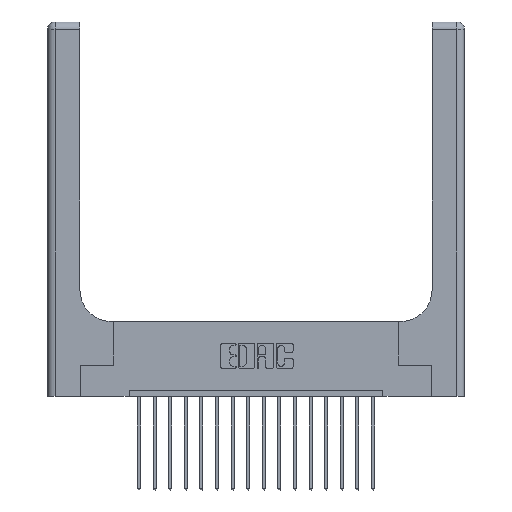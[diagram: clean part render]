
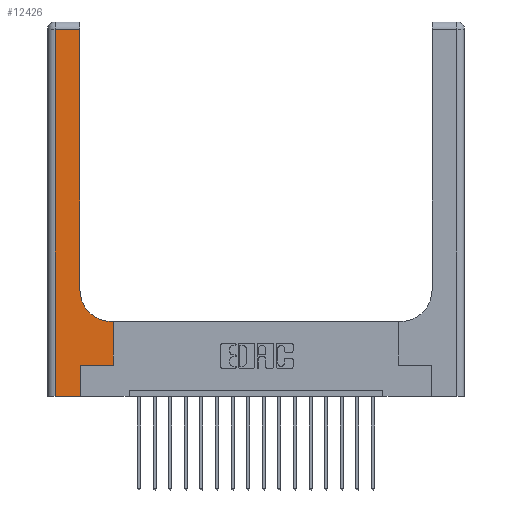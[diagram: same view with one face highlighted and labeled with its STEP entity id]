
A CAD part, top view. The second image highlights one B-rep face of the part: STEP entity #12426.
In plain terms, the highlighted planar face has unit normal (0, 0, 1).
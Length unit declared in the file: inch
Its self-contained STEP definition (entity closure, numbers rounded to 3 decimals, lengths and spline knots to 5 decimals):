
#33 = VERTEX_POINT ( 'NONE', #1274 ) ;
#630 = DIRECTION ( 'NONE',  ( 0., 1., 0. ) ) ;
#940 = CARTESIAN_POINT ( 'NONE',  ( 0., 3., 0.37 ) ) ;
#1027 = EDGE_CURVE ( 'NONE', #11194, #11451, #1147, .T. ) ;
#1114 = DIRECTION ( 'NONE',  ( 0., 0., -1. ) ) ;
#1147 = LINE ( 'NONE', #8319, #17055 ) ;
#1274 = CARTESIAN_POINT ( 'NONE',  ( 0.528, 0.25, 0.37 ) ) ;
#1465 = CARTESIAN_POINT ( 'NONE',  ( 0.26, 0.6, 0.37 ) ) ;
#2452 = CARTESIAN_POINT ( 'NONE',  ( 0., 2.94, 0.37 ) ) ;
#2716 = ORIENTED_EDGE ( 'NONE', *, *, #4528, .T. ) ;
#3348 = AXIS2_PLACEMENT_3D ( 'NONE', #3932, #9859, #8403 ) ;
#3686 = EDGE_CURVE ( 'NONE', #17438, #12277, #15070, .T. ) ;
#3751 = CARTESIAN_POINT ( 'NONE',  ( 0.265, 0.25, 0.37 ) ) ;
#3831 = VECTOR ( 'NONE', #13828, 39.37008 ) ;
#3932 = CARTESIAN_POINT ( 'NONE',  ( 0.51, 0.85, 0.37 ) ) ;
#4528 = EDGE_CURVE ( 'NONE', #11451, #11347, #7213, .T. ) ;
#4655 = CARTESIAN_POINT ( 'NONE',  ( 0.265, 0., 0.37 ) ) ;
#5297 = CARTESIAN_POINT ( 'NONE',  ( 0.26, 3., 0.37 ) ) ;
#5435 = LINE ( 'NONE', #2452, #6030 ) ;
#5546 = FACE_OUTER_BOUND ( 'NONE', #7995, .T. ) ;
#5766 = DIRECTION ( 'NONE',  ( 1., 0., 0. ) ) ;
#5840 = ORIENTED_EDGE ( 'NONE', *, *, #18674, .T. ) ;
#6030 = VECTOR ( 'NONE', #10095, 39.37008 ) ;
#6443 = EDGE_CURVE ( 'NONE', #11347, #12802, #13176, .T. ) ;
#6782 = ORIENTED_EDGE ( 'NONE', *, *, #14539, .T. ) ;
#7085 = DIRECTION ( 'NONE',  ( -1., 0., 0. ) ) ;
#7105 = CARTESIAN_POINT ( 'NONE',  ( 0.528, 0.6, 0.37 ) ) ;
#7213 = LINE ( 'NONE', #18970, #13545 ) ;
#7329 = CARTESIAN_POINT ( 'NONE',  ( 0.265, 0., 0.37 ) ) ;
#7671 = DIRECTION ( 'NONE',  ( 1., 0., 0. ) ) ;
#7859 = LINE ( 'NONE', #15298, #17080 ) ;
#7995 = EDGE_LOOP ( 'NONE', ( #12732, #17439, #17135, #2716, #16344, #5840, #6782, #9840, #17168 ) ) ;
#8319 = CARTESIAN_POINT ( 'NONE',  ( 0.06, 3., 0.37 ) ) ;
#8403 = DIRECTION ( 'NONE',  ( 1., 0., 0. ) ) ;
#8407 = DIRECTION ( 'NONE',  ( 0., -1., 0. ) ) ;
#9840 = ORIENTED_EDGE ( 'NONE', *, *, #13512, .T. ) ;
#9859 = DIRECTION ( 'NONE',  ( 0., 0., -1. ) ) ;
#10095 = DIRECTION ( 'NONE',  ( -1., 0., 0. ) ) ;
#10264 = VECTOR ( 'NONE', #7085, 39.37008 ) ;
#10365 = DIRECTION ( 'NONE',  ( 0., 1., 0. ) ) ;
#10501 = VERTEX_POINT ( 'NONE', #17712 ) ;
#10522 = VERTEX_POINT ( 'NONE', #7105 ) ;
#10687 = VECTOR ( 'NONE', #7671, 39.37008 ) ;
#11194 = VERTEX_POINT ( 'NONE', #17579 ) ;
#11347 = VERTEX_POINT ( 'NONE', #7329 ) ;
#11451 = VERTEX_POINT ( 'NONE', #11456 ) ;
#11456 = CARTESIAN_POINT ( 'NONE',  ( 0.06, 0., 0.37 ) ) ;
#12277 = VERTEX_POINT ( 'NONE', #16855 ) ;
#12426 = ADVANCED_FACE ( 'NONE', ( #5546 ), #18675, .F. ) ;
#12732 = ORIENTED_EDGE ( 'NONE', *, *, #16844, .T. ) ;
#12802 = VERTEX_POINT ( 'NONE', #3751 ) ;
#13176 = LINE ( 'NONE', #4655, #13412 ) ;
#13408 = CARTESIAN_POINT ( 'NONE',  ( 0.265, 0.25, 0.37 ) ) ;
#13412 = VECTOR ( 'NONE', #10365, 39.37008 ) ;
#13512 = EDGE_CURVE ( 'NONE', #10522, #17438, #14707, .T. ) ;
#13545 = VECTOR ( 'NONE', #5766, 39.37008 ) ;
#13828 = DIRECTION ( 'NONE',  ( 0., 1., 0. ) ) ;
#14114 = LINE ( 'NONE', #5297, #3831 ) ;
#14539 = EDGE_CURVE ( 'NONE', #33, #10522, #7859, .T. ) ;
#14707 = LINE ( 'NONE', #1465, #10264 ) ;
#15070 = CIRCLE ( 'NONE', #3348, 0.25 ) ;
#15298 = CARTESIAN_POINT ( 'NONE',  ( 0.528, 0.25, 0.37 ) ) ;
#15459 = AXIS2_PLACEMENT_3D ( 'NONE', #940, #1114, #15761 ) ;
#15761 = DIRECTION ( 'NONE',  ( -1., 0., 0. ) ) ;
#16344 = ORIENTED_EDGE ( 'NONE', *, *, #6443, .T. ) ;
#16844 = EDGE_CURVE ( 'NONE', #12277, #10501, #14114, .T. ) ;
#16855 = CARTESIAN_POINT ( 'NONE',  ( 0.26, 0.85, 0.37 ) ) ;
#17055 = VECTOR ( 'NONE', #8407, 39.37008 ) ;
#17080 = VECTOR ( 'NONE', #630, 39.37008 ) ;
#17135 = ORIENTED_EDGE ( 'NONE', *, *, #1027, .T. ) ;
#17168 = ORIENTED_EDGE ( 'NONE', *, *, #3686, .T. ) ;
#17438 = VERTEX_POINT ( 'NONE', #18685 ) ;
#17439 = ORIENTED_EDGE ( 'NONE', *, *, #18965, .T. ) ;
#17579 = CARTESIAN_POINT ( 'NONE',  ( 0.06, 2.94, 0.37 ) ) ;
#17712 = CARTESIAN_POINT ( 'NONE',  ( 0.26, 2.94, 0.37 ) ) ;
#18004 = LINE ( 'NONE', #13408, #10687 ) ;
#18674 = EDGE_CURVE ( 'NONE', #12802, #33, #18004, .T. ) ;
#18675 = PLANE ( 'NONE',  #15459 ) ;
#18685 = CARTESIAN_POINT ( 'NONE',  ( 0.51, 0.6, 0.37 ) ) ;
#18965 = EDGE_CURVE ( 'NONE', #10501, #11194, #5435, .T. ) ;
#18970 = CARTESIAN_POINT ( 'NONE',  ( 0., 0., 0.37 ) ) ;
